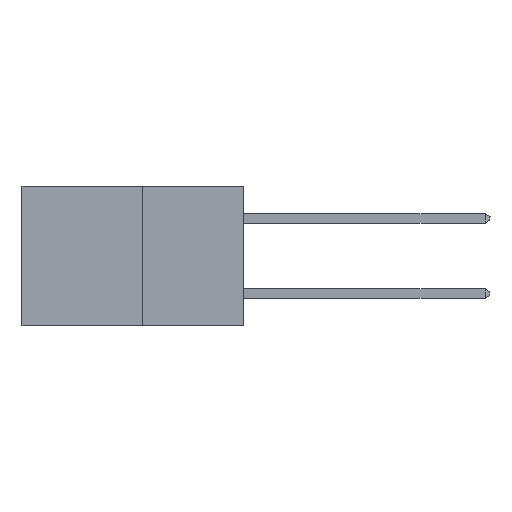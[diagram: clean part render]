
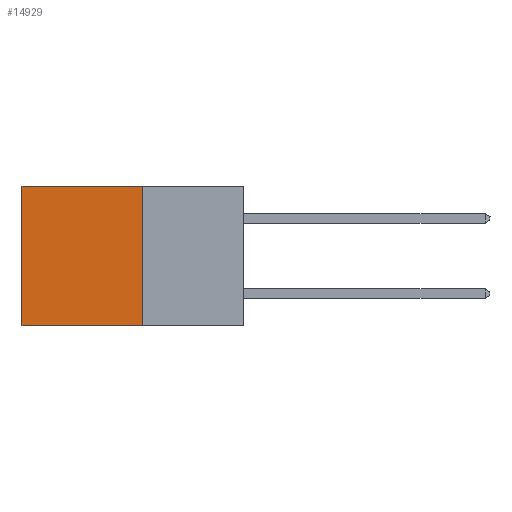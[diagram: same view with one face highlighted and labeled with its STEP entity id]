
A CAD part, left-side view. The second image highlights one B-rep face of the part: STEP entity #14929.
In plain terms, the highlighted planar face has unit normal (-1, 0, 0).
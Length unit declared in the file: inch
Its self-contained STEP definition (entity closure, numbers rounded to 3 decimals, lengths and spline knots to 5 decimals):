
#249 = FACE_OUTER_BOUND ( 'NONE', #13875, .T. ) ;
#1123 = VERTEX_POINT ( 'NONE', #4215 ) ;
#1269 = VECTOR ( 'NONE', #1553, 39.37008 ) ;
#1553 = DIRECTION ( 'NONE',  ( 0., 0., -1. ) ) ;
#1836 = ORIENTED_EDGE ( 'NONE', *, *, #12376, .T. ) ;
#1853 = CARTESIAN_POINT ( 'NONE',  ( 0.277, 0.59, 0. ) ) ;
#1883 = EDGE_CURVE ( 'NONE', #10761, #1123, #8481, .T. ) ;
#2128 = ORIENTED_EDGE ( 'NONE', *, *, #6435, .T. ) ;
#2994 = CARTESIAN_POINT ( 'NONE',  ( 0.277, 0.27, -0.37 ) ) ;
#3034 = DIRECTION ( 'NONE',  ( 1., 0., 0. ) ) ;
#4215 = CARTESIAN_POINT ( 'NONE',  ( 0.277, 0.59, -0.37 ) ) ;
#4286 = DIRECTION ( 'NONE',  ( 0., 1., 0. ) ) ;
#4501 = ORIENTED_EDGE ( 'NONE', *, *, #1883, .F. ) ;
#5141 = VECTOR ( 'NONE', #12862, 39.37008 ) ;
#6435 = EDGE_CURVE ( 'NONE', #17854, #15892, #11856, .T. ) ;
#7881 = CARTESIAN_POINT ( 'NONE',  ( 0.277, 0.59, -0.37 ) ) ;
#8435 = LINE ( 'NONE', #2994, #1269 ) ;
#8481 = LINE ( 'NONE', #13009, #5141 ) ;
#10019 = VECTOR ( 'NONE', #14987, 39.37008 ) ;
#10761 = VERTEX_POINT ( 'NONE', #14916 ) ;
#11556 = CARTESIAN_POINT ( 'NONE',  ( 0.277, 0.27, -0.37 ) ) ;
#11856 = LINE ( 'NONE', #15628, #15609 ) ;
#12376 = EDGE_CURVE ( 'NONE', #15892, #1123, #13780, .T. ) ;
#12862 = DIRECTION ( 'NONE',  ( 0., 1., 0. ) ) ;
#12991 = DIRECTION ( 'NONE',  ( 0., 0., -1. ) ) ;
#13009 = CARTESIAN_POINT ( 'NONE',  ( 0.277, 0.27, -0.37 ) ) ;
#13518 = ORIENTED_EDGE ( 'NONE', *, *, #17767, .F. ) ;
#13780 = LINE ( 'NONE', #7881, #10019 ) ;
#13875 = EDGE_LOOP ( 'NONE', ( #1836, #4501, #13518, #2128 ) ) ;
#14307 = AXIS2_PLACEMENT_3D ( 'NONE', #11556, #3034, #12991 ) ;
#14916 = CARTESIAN_POINT ( 'NONE',  ( 0.277, 0.27, -0.37 ) ) ;
#14929 = ADVANCED_FACE ( 'NONE', ( #249 ), #17137, .F. ) ;
#14987 = DIRECTION ( 'NONE',  ( 0., 0., -1. ) ) ;
#15609 = VECTOR ( 'NONE', #4286, 39.37008 ) ;
#15628 = CARTESIAN_POINT ( 'NONE',  ( 0.277, 0.27, 0. ) ) ;
#15892 = VERTEX_POINT ( 'NONE', #1853 ) ;
#17137 = PLANE ( 'NONE',  #14307 ) ;
#17327 = CARTESIAN_POINT ( 'NONE',  ( 0.277, 0.27, 0. ) ) ;
#17767 = EDGE_CURVE ( 'NONE', #17854, #10761, #8435, .T. ) ;
#17854 = VERTEX_POINT ( 'NONE', #17327 ) ;
